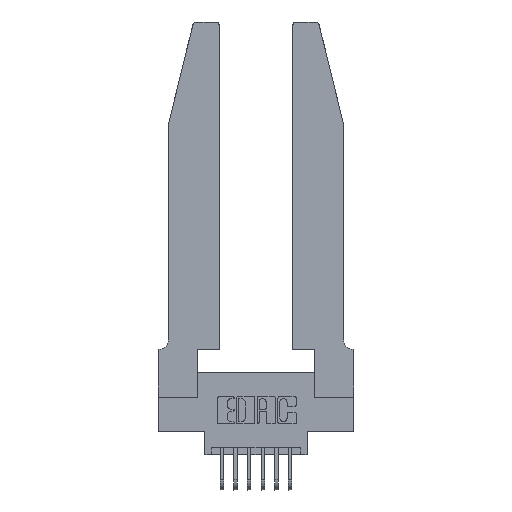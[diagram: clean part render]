
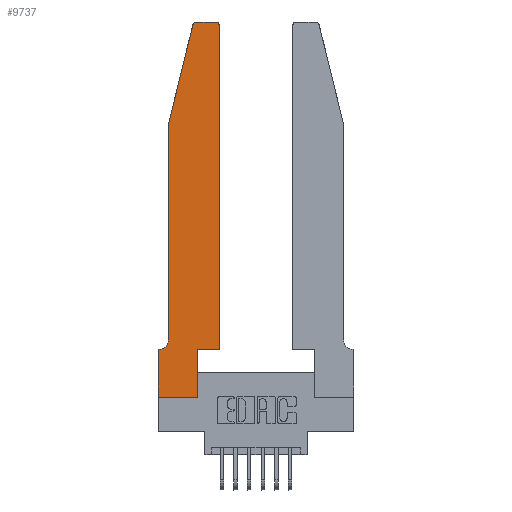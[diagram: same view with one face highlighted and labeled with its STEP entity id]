
A CAD part, top view. The second image highlights one B-rep face of the part: STEP entity #9737.
In plain terms, the highlighted planar face has unit normal (0, 0, 1).
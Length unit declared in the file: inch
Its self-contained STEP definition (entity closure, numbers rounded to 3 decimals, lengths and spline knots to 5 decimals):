
#18 = VERTEX_POINT ( 'NONE', #2326 ) ;
#98 = DIRECTION ( 'NONE',  ( 0., 1., 0. ) ) ;
#178 = CIRCLE ( 'NONE', #4159, 0.03 ) ;
#297 = FACE_OUTER_BOUND ( 'NONE', #11282, .T. ) ;
#468 = CIRCLE ( 'NONE', #10096, 0.03 ) ;
#537 = DIRECTION ( 'NONE',  ( 0., 1., 0. ) ) ;
#600 = CARTESIAN_POINT ( 'NONE',  ( 0.0055, 0.42, 0.37 ) ) ;
#602 = VERTEX_POINT ( 'NONE', #6554 ) ;
#654 = DIRECTION ( 'NONE',  ( 0., 0., -1. ) ) ;
#700 = CARTESIAN_POINT ( 'NONE',  ( 0.0055, 0.35, 0.37 ) ) ;
#790 = LINE ( 'NONE', #6348, #3118 ) ;
#796 = EDGE_CURVE ( 'NONE', #3154, #1894, #4220, .T. ) ;
#851 = VECTOR ( 'NONE', #10595, 39.37008 ) ;
#905 = CARTESIAN_POINT ( 'NONE',  ( 0.4205, 2.72, 0.37 ) ) ;
#1171 = CARTESIAN_POINT ( 'NONE',  ( 0., 0., 0.37 ) ) ;
#1478 = CARTESIAN_POINT ( 'NONE',  ( 0.284, 2.75, 0.37 ) ) ;
#1836 = ORIENTED_EDGE ( 'NONE', *, *, #2014, .T. ) ;
#1894 = VERTEX_POINT ( 'NONE', #1478 ) ;
#2014 = EDGE_CURVE ( 'NONE', #18, #9499, #5369, .T. ) ;
#2017 = VERTEX_POINT ( 'NONE', #4493 ) ;
#2068 = DIRECTION ( 'NONE',  ( 1., 0., 0. ) ) ;
#2114 = PLANE ( 'NONE',  #4125 ) ;
#2138 = VECTOR ( 'NONE', #5908, 39.37008 ) ;
#2148 = ORIENTED_EDGE ( 'NONE', *, *, #6553, .T. ) ;
#2215 = DIRECTION ( 'NONE',  ( 1., 0., 0. ) ) ;
#2326 = CARTESIAN_POINT ( 'NONE',  ( 0.0755, 0.42, 0.37 ) ) ;
#2400 = VECTOR ( 'NONE', #12839, 39.37008 ) ;
#2426 = CARTESIAN_POINT ( 'NONE',  ( 0.2865, 0.35, 0.37 ) ) ;
#2434 = CARTESIAN_POINT ( 'NONE',  ( 0.0755, 2., 0.37 ) ) ;
#2498 = ORIENTED_EDGE ( 'NONE', *, *, #9409, .T. ) ;
#3002 = DIRECTION ( 'NONE',  ( -1., 0., 0. ) ) ;
#3118 = VECTOR ( 'NONE', #3002, 39.37008 ) ;
#3154 = VERTEX_POINT ( 'NONE', #5813 ) ;
#3294 = EDGE_CURVE ( 'NONE', #8855, #11152, #14253, .T. ) ;
#3671 = CARTESIAN_POINT ( 'NONE',  ( 0., 0., 0.37 ) ) ;
#3989 = CARTESIAN_POINT ( 'NONE',  ( 0.0755, 2., 0.37 ) ) ;
#4026 = ORIENTED_EDGE ( 'NONE', *, *, #6743, .T. ) ;
#4033 = VECTOR ( 'NONE', #9261, 39.37008 ) ;
#4125 = AXIS2_PLACEMENT_3D ( 'NONE', #7701, #8804, #2215 ) ;
#4159 = AXIS2_PLACEMENT_3D ( 'NONE', #905, #8670, #2068 ) ;
#4191 = DIRECTION ( 'NONE',  ( -1., 0., 0. ) ) ;
#4219 = VECTOR ( 'NONE', #537, 39.37008 ) ;
#4220 = LINE ( 'NONE', #6117, #851 ) ;
#4493 = CARTESIAN_POINT ( 'NONE',  ( 0.25487, 2.72718, 0.37 ) ) ;
#4511 = VECTOR ( 'NONE', #98, 39.37008 ) ;
#4572 = CARTESIAN_POINT ( 'NONE',  ( 0.2865, 0.35, 0.37 ) ) ;
#4648 = ORIENTED_EDGE ( 'NONE', *, *, #5734, .T. ) ;
#4776 = CARTESIAN_POINT ( 'NONE',  ( 0., 0., 0.37 ) ) ;
#4840 = CARTESIAN_POINT ( 'NONE',  ( 0.0755, 2., 0.37 ) ) ;
#5369 = CIRCLE ( 'NONE', #6330, 0.07 ) ;
#5497 = DIRECTION ( 'NONE',  ( 1., 0., 0. ) ) ;
#5734 = EDGE_CURVE ( 'NONE', #11152, #13585, #7995, .T. ) ;
#5813 = CARTESIAN_POINT ( 'NONE',  ( 0.4205, 2.75, 0.37 ) ) ;
#5908 = DIRECTION ( 'NONE',  ( 1., 0., 0. ) ) ;
#5983 = CARTESIAN_POINT ( 'NONE',  ( 0.4505, 2.72, 0.37 ) ) ;
#6117 = CARTESIAN_POINT ( 'NONE',  ( 0.2605, 2.75, 0.37 ) ) ;
#6230 = ORIENTED_EDGE ( 'NONE', *, *, #11989, .T. ) ;
#6311 = CARTESIAN_POINT ( 'NONE',  ( 0., 0.35, 0.37 ) ) ;
#6330 = AXIS2_PLACEMENT_3D ( 'NONE', #600, #654, #4191 ) ;
#6348 = CARTESIAN_POINT ( 'NONE',  ( 0.0755, 0.35, 0.37 ) ) ;
#6553 = EDGE_CURVE ( 'NONE', #1894, #2017, #468, .T. ) ;
#6554 = CARTESIAN_POINT ( 'NONE',  ( 0.4505, 0.35, 0.37 ) ) ;
#6639 = ORIENTED_EDGE ( 'NONE', *, *, #11441, .T. ) ;
#6700 = CARTESIAN_POINT ( 'NONE',  ( 0.284, 2.72, 0.37 ) ) ;
#6736 = VERTEX_POINT ( 'NONE', #5983 ) ;
#6743 = EDGE_CURVE ( 'NONE', #2017, #8545, #6942, .T. ) ;
#6942 = LINE ( 'NONE', #4840, #4033 ) ;
#7133 = LINE ( 'NONE', #13832, #4219 ) ;
#7439 = LINE ( 'NONE', #4572, #4511 ) ;
#7701 = CARTESIAN_POINT ( 'NONE',  ( 0., 0.35, 0.37 ) ) ;
#7733 = EDGE_CURVE ( 'NONE', #13585, #11753, #7439, .T. ) ;
#7781 = DIRECTION ( 'NONE',  ( 1., 0., 0. ) ) ;
#7866 = VECTOR ( 'NONE', #5497, 39.37008 ) ;
#7995 = LINE ( 'NONE', #3671, #2138 ) ;
#8201 = LINE ( 'NONE', #13217, #7866 ) ;
#8241 = LINE ( 'NONE', #3989, #2400 ) ;
#8545 = VERTEX_POINT ( 'NONE', #2434 ) ;
#8670 = DIRECTION ( 'NONE',  ( 0., 0., 1. ) ) ;
#8804 = DIRECTION ( 'NONE',  ( 0., 0., 1. ) ) ;
#8855 = VERTEX_POINT ( 'NONE', #6311 ) ;
#8921 = ORIENTED_EDGE ( 'NONE', *, *, #13468, .T. ) ;
#9261 = DIRECTION ( 'NONE',  ( -0.239, -0.971, 0. ) ) ;
#9409 = EDGE_CURVE ( 'NONE', #602, #6736, #7133, .T. ) ;
#9499 = VERTEX_POINT ( 'NONE', #700 ) ;
#9737 = ADVANCED_FACE ( 'NONE', ( #297 ), #2114, .T. ) ;
#10096 = AXIS2_PLACEMENT_3D ( 'NONE', #6700, #14322, #7781 ) ;
#10113 = CARTESIAN_POINT ( 'NONE',  ( 0.2865, 0., 0.37 ) ) ;
#10381 = ORIENTED_EDGE ( 'NONE', *, *, #7733, .T. ) ;
#10595 = DIRECTION ( 'NONE',  ( -1., 0., 0. ) ) ;
#10862 = ORIENTED_EDGE ( 'NONE', *, *, #796, .T. ) ;
#11152 = VERTEX_POINT ( 'NONE', #4776 ) ;
#11282 = EDGE_LOOP ( 'NONE', ( #10862, #2148, #4026, #6230, #1836, #6639, #11840, #4648, #10381, #8921, #2498, #12072 ) ) ;
#11441 = EDGE_CURVE ( 'NONE', #9499, #8855, #790, .T. ) ;
#11753 = VERTEX_POINT ( 'NONE', #2426 ) ;
#11840 = ORIENTED_EDGE ( 'NONE', *, *, #3294, .T. ) ;
#11989 = EDGE_CURVE ( 'NONE', #8545, #18, #8241, .T. ) ;
#12072 = ORIENTED_EDGE ( 'NONE', *, *, #14031, .T. ) ;
#12327 = DIRECTION ( 'NONE',  ( 0., -1., 0. ) ) ;
#12839 = DIRECTION ( 'NONE',  ( 0., -1., 0. ) ) ;
#13217 = CARTESIAN_POINT ( 'NONE',  ( 0.4505, 0.35, 0.37 ) ) ;
#13468 = EDGE_CURVE ( 'NONE', #11753, #602, #8201, .T. ) ;
#13585 = VERTEX_POINT ( 'NONE', #10113 ) ;
#13600 = VECTOR ( 'NONE', #12327, 39.37008 ) ;
#13832 = CARTESIAN_POINT ( 'NONE',  ( 0.4505, 0.35, 0.37 ) ) ;
#14031 = EDGE_CURVE ( 'NONE', #6736, #3154, #178, .T. ) ;
#14253 = LINE ( 'NONE', #1171, #13600 ) ;
#14322 = DIRECTION ( 'NONE',  ( 0., 0., 1. ) ) ;
